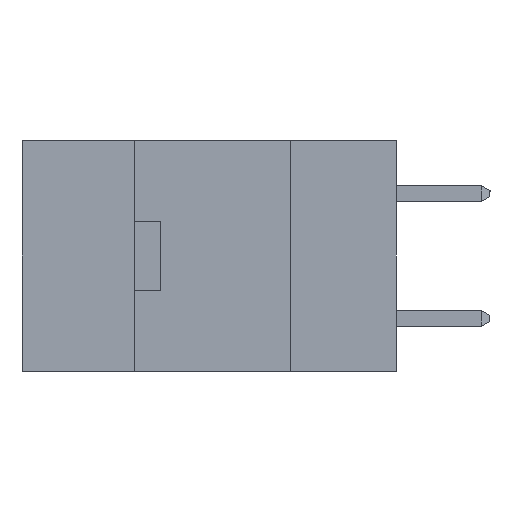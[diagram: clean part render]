
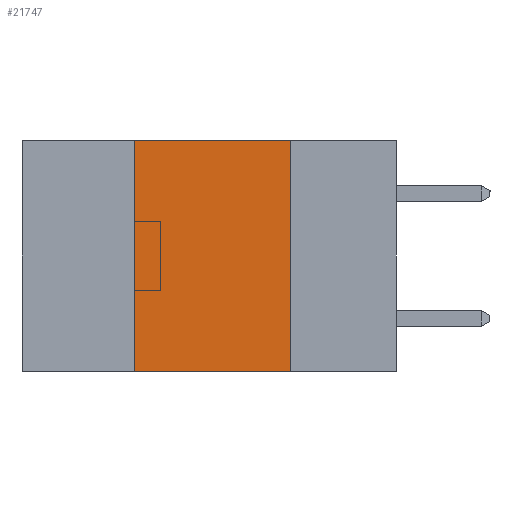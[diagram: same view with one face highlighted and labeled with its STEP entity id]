
A CAD part, left-side view. The second image highlights one B-rep face of the part: STEP entity #21747.
In plain terms, the highlighted planar face has unit normal (-1, 0, 0).
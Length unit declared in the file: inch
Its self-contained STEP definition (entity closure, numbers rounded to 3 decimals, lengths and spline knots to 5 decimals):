
#225 = DIRECTION ( 'NONE',  ( 0., 0., -1. ) ) ;
#372 = CARTESIAN_POINT ( 'NONE',  ( 0., 0.42, -0.37 ) ) ;
#410 = CARTESIAN_POINT ( 'NONE',  ( 0., 0.6, 0. ) ) ;
#799 = DIRECTION ( 'NONE',  ( 0., 0., 1. ) ) ;
#1287 = EDGE_LOOP ( 'NONE', ( #21694, #2847, #3125, #8050 ) ) ;
#2101 = CARTESIAN_POINT ( 'NONE',  ( 0., 0.6, 0. ) ) ;
#2847 = ORIENTED_EDGE ( 'NONE', *, *, #14008, .F. ) ;
#2895 = EDGE_CURVE ( 'NONE', #16526, #14108, #8557, .T. ) ;
#3125 = ORIENTED_EDGE ( 'NONE', *, *, #15034, .F. ) ;
#5463 = CARTESIAN_POINT ( 'NONE',  ( 0., 0.42, -0.37 ) ) ;
#5842 = CARTESIAN_POINT ( 'NONE',  ( 0., 0.42, 0. ) ) ;
#8050 = ORIENTED_EDGE ( 'NONE', *, *, #24386, .T. ) ;
#8464 = VERTEX_POINT ( 'NONE', #372 ) ;
#8557 = LINE ( 'NONE', #15294, #17690 ) ;
#9033 = DIRECTION ( 'NONE',  ( 0., -1., 0. ) ) ;
#9286 = VECTOR ( 'NONE', #9033, 39.37008 ) ;
#9315 = DIRECTION ( 'NONE',  ( 1., 0., 0. ) ) ;
#13132 = DIRECTION ( 'NONE',  ( 0., 0., -1. ) ) ;
#13196 = DIRECTION ( 'NONE',  ( 0., -1., 0. ) ) ;
#13810 = VECTOR ( 'NONE', #13196, 39.37008 ) ;
#14008 = EDGE_CURVE ( 'NONE', #17553, #16526, #26820, .T. ) ;
#14108 = VERTEX_POINT ( 'NONE', #27960 ) ;
#15034 = EDGE_CURVE ( 'NONE', #8464, #17553, #20872, .T. ) ;
#15294 = CARTESIAN_POINT ( 'NONE',  ( 0., 0.17, -0.37 ) ) ;
#15937 = AXIS2_PLACEMENT_3D ( 'NONE', #410, #9315, #13132 ) ;
#16526 = VERTEX_POINT ( 'NONE', #24088 ) ;
#16654 = VECTOR ( 'NONE', #799, 39.37008 ) ;
#17553 = VERTEX_POINT ( 'NONE', #5842 ) ;
#17690 = VECTOR ( 'NONE', #225, 39.37008 ) ;
#20346 = LINE ( 'NONE', #27346, #9286 ) ;
#20472 = PLANE ( 'NONE',  #15937 ) ;
#20872 = LINE ( 'NONE', #5463, #16654 ) ;
#21694 = ORIENTED_EDGE ( 'NONE', *, *, #2895, .F. ) ;
#21747 = ADVANCED_FACE ( 'NONE', ( #24553 ), #20472, .F. ) ;
#24088 = CARTESIAN_POINT ( 'NONE',  ( 0., 0.17, 0. ) ) ;
#24386 = EDGE_CURVE ( 'NONE', #8464, #14108, #20346, .T. ) ;
#24553 = FACE_OUTER_BOUND ( 'NONE', #1287, .T. ) ;
#26820 = LINE ( 'NONE', #2101, #13810 ) ;
#27346 = CARTESIAN_POINT ( 'NONE',  ( 0., 0.6, -0.37 ) ) ;
#27960 = CARTESIAN_POINT ( 'NONE',  ( 0., 0.17, -0.37 ) ) ;
